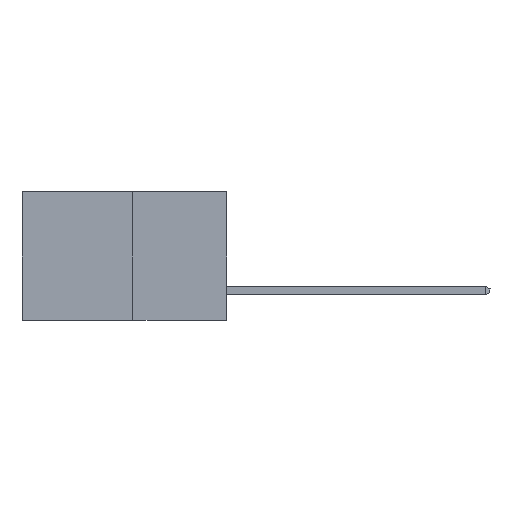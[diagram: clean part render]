
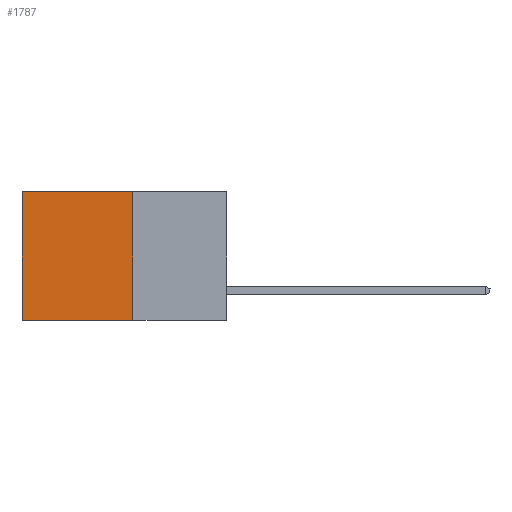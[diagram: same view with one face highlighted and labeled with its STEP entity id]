
A CAD part, left-side view. The second image highlights one B-rep face of the part: STEP entity #1787.
In plain terms, the highlighted planar face has unit normal (-1, 0, 0).
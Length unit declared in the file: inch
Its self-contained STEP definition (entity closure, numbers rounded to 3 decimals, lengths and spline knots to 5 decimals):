
#588 = CARTESIAN_POINT ( 'NONE',  ( 0.277, 0.59, -0.37 ) ) ;
#725 = EDGE_CURVE ( 'NONE', #4912, #3971, #7842, .T. ) ;
#755 = EDGE_CURVE ( 'NONE', #5572, #14722, #13196, .T. ) ;
#963 = CARTESIAN_POINT ( 'NONE',  ( 0.277, 0.27, 0. ) ) ;
#1036 = FACE_OUTER_BOUND ( 'NONE', #9909, .T. ) ;
#1787 = ADVANCED_FACE ( 'NONE', ( #1036 ), #8605, .F. ) ;
#2125 = CARTESIAN_POINT ( 'NONE',  ( 0.277, 0.59, 0. ) ) ;
#2127 = DIRECTION ( 'NONE',  ( 0., 1., 0. ) ) ;
#3026 = ORIENTED_EDGE ( 'NONE', *, *, #755, .F. ) ;
#3857 = EDGE_CURVE ( 'NONE', #14722, #3971, #7754, .T. ) ;
#3971 = VERTEX_POINT ( 'NONE', #12940 ) ;
#4351 = DIRECTION ( 'NONE',  ( 0., 0., -1. ) ) ;
#4816 = AXIS2_PLACEMENT_3D ( 'NONE', #7711, #9371, #7775 ) ;
#4902 = CARTESIAN_POINT ( 'NONE',  ( 0.277, 0.27, -0.37 ) ) ;
#4912 = VERTEX_POINT ( 'NONE', #2125 ) ;
#5045 = CARTESIAN_POINT ( 'NONE',  ( 0.277, 0.27, 0. ) ) ;
#5572 = VERTEX_POINT ( 'NONE', #5045 ) ;
#5863 = LINE ( 'NONE', #963, #11595 ) ;
#7034 = VECTOR ( 'NONE', #14400, 39.37008 ) ;
#7572 = DIRECTION ( 'NONE',  ( 0., 0., -1. ) ) ;
#7711 = CARTESIAN_POINT ( 'NONE',  ( 0.277, 0.27, -0.37 ) ) ;
#7754 = LINE ( 'NONE', #14447, #7034 ) ;
#7775 = DIRECTION ( 'NONE',  ( 0., 0., -1. ) ) ;
#7842 = LINE ( 'NONE', #588, #14312 ) ;
#8605 = PLANE ( 'NONE',  #4816 ) ;
#9371 = DIRECTION ( 'NONE',  ( 1., 0., 0. ) ) ;
#9909 = EDGE_LOOP ( 'NONE', ( #11963, #15024, #3026, #12324 ) ) ;
#9979 = CARTESIAN_POINT ( 'NONE',  ( 0.277, 0.27, -0.37 ) ) ;
#10514 = VECTOR ( 'NONE', #4351, 39.37008 ) ;
#11595 = VECTOR ( 'NONE', #2127, 39.37008 ) ;
#11963 = ORIENTED_EDGE ( 'NONE', *, *, #725, .T. ) ;
#12324 = ORIENTED_EDGE ( 'NONE', *, *, #14159, .T. ) ;
#12940 = CARTESIAN_POINT ( 'NONE',  ( 0.277, 0.59, -0.37 ) ) ;
#13196 = LINE ( 'NONE', #4902, #10514 ) ;
#14159 = EDGE_CURVE ( 'NONE', #5572, #4912, #5863, .T. ) ;
#14312 = VECTOR ( 'NONE', #7572, 39.37008 ) ;
#14400 = DIRECTION ( 'NONE',  ( 0., 1., 0. ) ) ;
#14447 = CARTESIAN_POINT ( 'NONE',  ( 0.277, 0.27, -0.37 ) ) ;
#14722 = VERTEX_POINT ( 'NONE', #9979 ) ;
#15024 = ORIENTED_EDGE ( 'NONE', *, *, #3857, .F. ) ;
